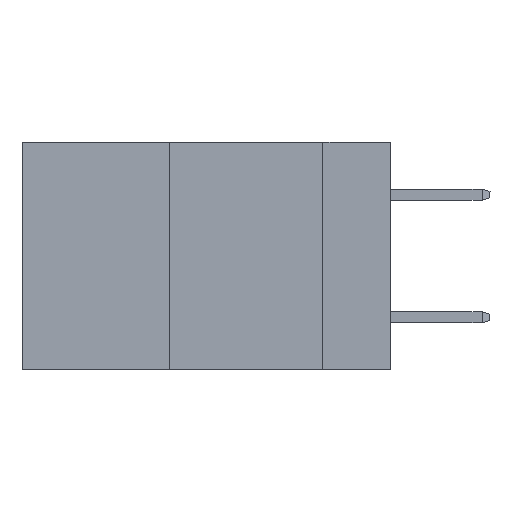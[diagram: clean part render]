
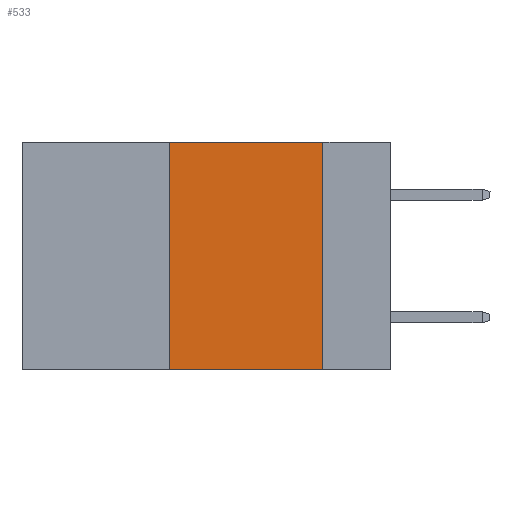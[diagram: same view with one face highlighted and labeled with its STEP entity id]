
A CAD part, left-side view. The second image highlights one B-rep face of the part: STEP entity #533.
In plain terms, the highlighted planar face has unit normal (-1, 0, 0).
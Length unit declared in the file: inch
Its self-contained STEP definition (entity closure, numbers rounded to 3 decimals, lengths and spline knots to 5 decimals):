
#11 = LINE ( 'NONE', #14569, #17025 ) ;
#533 = ADVANCED_FACE ( 'NONE', ( #19637 ), #4297, .F. ) ;
#782 = CARTESIAN_POINT ( 'NONE',  ( 0., 0.36, 0. ) ) ;
#1374 = ORIENTED_EDGE ( 'NONE', *, *, #13289, .F. ) ;
#1953 = VERTEX_POINT ( 'NONE', #782 ) ;
#2380 = DIRECTION ( 'NONE',  ( 0., 0., 1. ) ) ;
#3103 = ORIENTED_EDGE ( 'NONE', *, *, #9467, .F. ) ;
#3487 = CARTESIAN_POINT ( 'NONE',  ( 0., 0.36, -0.37 ) ) ;
#3851 = CARTESIAN_POINT ( 'NONE',  ( 0., 0.6, 0. ) ) ;
#3913 = DIRECTION ( 'NONE',  ( 0., 0., -1. ) ) ;
#4297 = PLANE ( 'NONE',  #21134 ) ;
#4386 = CARTESIAN_POINT ( 'NONE',  ( 0., 0.11, 0. ) ) ;
#4569 = DIRECTION ( 'NONE',  ( 0., -1., 0. ) ) ;
#6087 = VECTOR ( 'NONE', #13688, 39.37008 ) ;
#7769 = CARTESIAN_POINT ( 'NONE',  ( 0., 0.6, -0.37 ) ) ;
#9467 = EDGE_CURVE ( 'NONE', #1953, #11163, #14293, .T. ) ;
#10593 = CARTESIAN_POINT ( 'NONE',  ( 0., 0.36, 0. ) ) ;
#10902 = EDGE_LOOP ( 'NONE', ( #12654, #3103, #1374, #20730 ) ) ;
#11163 = VERTEX_POINT ( 'NONE', #4386 ) ;
#12654 = ORIENTED_EDGE ( 'NONE', *, *, #14837, .F. ) ;
#12811 = VERTEX_POINT ( 'NONE', #3487 ) ;
#13156 = LINE ( 'NONE', #10593, #20970 ) ;
#13289 = EDGE_CURVE ( 'NONE', #12811, #1953, #13156, .T. ) ;
#13688 = DIRECTION ( 'NONE',  ( 0., -1., 0. ) ) ;
#14293 = LINE ( 'NONE', #3851, #6087 ) ;
#14569 = CARTESIAN_POINT ( 'NONE',  ( 0., 0.11, 0. ) ) ;
#14837 = EDGE_CURVE ( 'NONE', #11163, #14952, #11, .T. ) ;
#14952 = VERTEX_POINT ( 'NONE', #18181 ) ;
#15798 = CARTESIAN_POINT ( 'NONE',  ( 0., 0.6, 0. ) ) ;
#16251 = VECTOR ( 'NONE', #4569, 39.37008 ) ;
#17025 = VECTOR ( 'NONE', #17899, 39.37008 ) ;
#17899 = DIRECTION ( 'NONE',  ( 0., 0., -1. ) ) ;
#18163 = EDGE_CURVE ( 'NONE', #12811, #14952, #20655, .T. ) ;
#18181 = CARTESIAN_POINT ( 'NONE',  ( 0., 0.11, -0.37 ) ) ;
#18970 = DIRECTION ( 'NONE',  ( 1., 0., 0. ) ) ;
#19637 = FACE_OUTER_BOUND ( 'NONE', #10902, .T. ) ;
#20655 = LINE ( 'NONE', #7769, #16251 ) ;
#20730 = ORIENTED_EDGE ( 'NONE', *, *, #18163, .T. ) ;
#20970 = VECTOR ( 'NONE', #2380, 39.37008 ) ;
#21134 = AXIS2_PLACEMENT_3D ( 'NONE', #15798, #18970, #3913 ) ;
